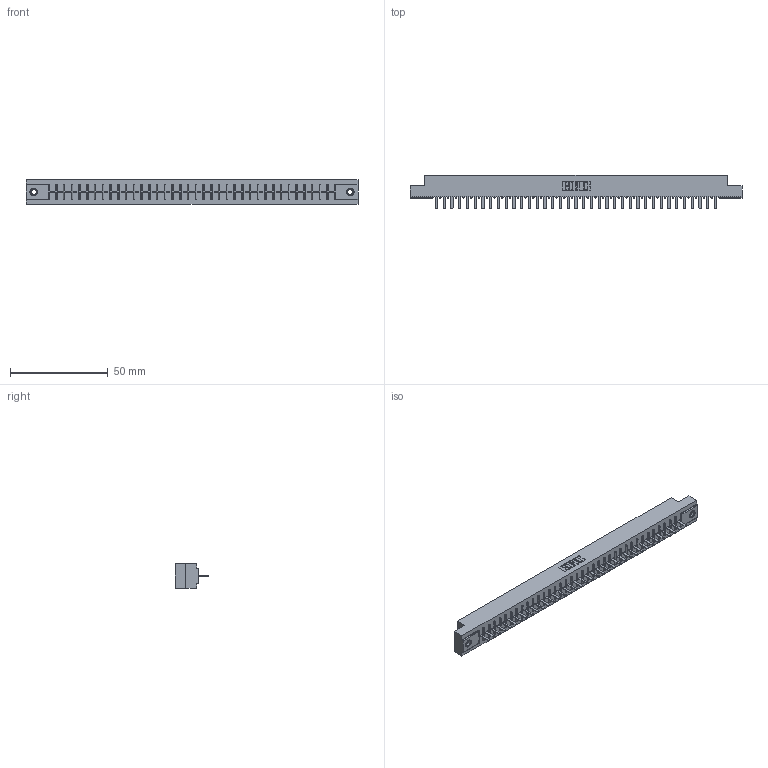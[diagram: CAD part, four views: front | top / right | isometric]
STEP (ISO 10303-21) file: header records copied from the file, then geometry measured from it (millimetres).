
FILE_DESCRIPTION (( 'STEP AP203' ), '1' );
FILE_NAME ('316-037-420-107.STEP', '2020-09-23T05:27:28', ( '' ), ( '' ), 'SwSTEP 2.0', 'SolidWorks 2020', '' );
FILE_SCHEMA (( 'CONFIG_CONTROL_DESIGN' ));
Length unit declared in the file: inch
Products named in the file (4): 306-290-001_120; 345-250-001_345-250-005-103; 316-037-420-107; 306 Part_.156 Dia
Assembly tree (40 placements, depth 2):
  316-037-420-107
    306 Part_.156 Dia
    306-290-001_120  x37
    345-250-001_345-250-005-103  x2
Bounding box: 169.62 x 17.12 x 12.7 mm (x, y, z)
Volume: 18711.4 mm3; surface area: 19189.9 mm2
Topology: 40 solids, 40 shells, 2766 faces, 7741 edges, 4954 vertices
Faces by surface type: plane 1839, cylinder 763, sphere 148, cone 12, torus 4
Entity records: 36293 total; most frequent: CARTESIAN_POINT 6073, ORIENTED_EDGE 6014, DIRECTION 5997, EDGE_CURVE 3007, LINE 2349, VECTOR 2349, VERTEX_POINT 1900, AXIS2_PLACEMENT_3D 1824
